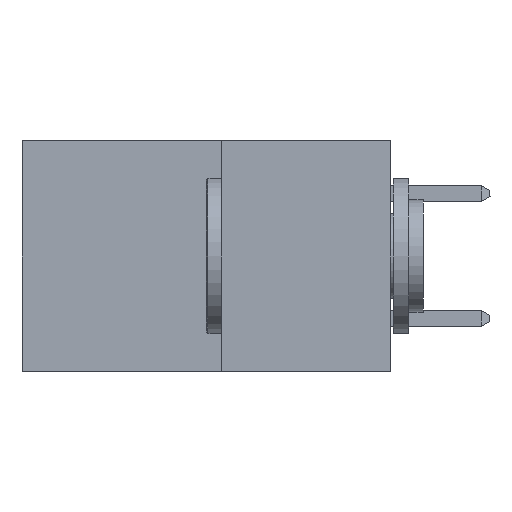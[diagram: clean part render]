
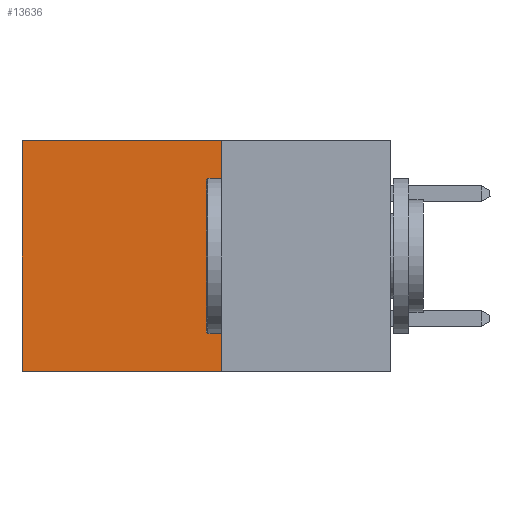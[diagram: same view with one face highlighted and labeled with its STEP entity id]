
A CAD part, left-side view. The second image highlights one B-rep face of the part: STEP entity #13636.
In plain terms, the highlighted planar face has unit normal (-1, 0, 0).
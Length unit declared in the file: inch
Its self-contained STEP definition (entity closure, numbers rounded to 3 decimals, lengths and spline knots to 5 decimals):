
#1156 = CARTESIAN_POINT ( 'NONE',  ( 0.277, 0.59, -0.37 ) ) ;
#1616 = FACE_OUTER_BOUND ( 'NONE', #6437, .T. ) ;
#2071 = CARTESIAN_POINT ( 'NONE',  ( 0.277, 0.27, -0.37 ) ) ;
#2269 = EDGE_CURVE ( 'NONE', #29836, #12502, #33518, .T. ) ;
#3433 = CARTESIAN_POINT ( 'NONE',  ( 0.277, 0.27, 0. ) ) ;
#3795 = ORIENTED_EDGE ( 'NONE', *, *, #24421, .F. ) ;
#4114 = CARTESIAN_POINT ( 'NONE',  ( 0.277, 0.27, -0.37 ) ) ;
#4438 = VECTOR ( 'NONE', #30401, 39.37008 ) ;
#4965 = VECTOR ( 'NONE', #28150, 39.37008 ) ;
#6162 = VECTOR ( 'NONE', #24502, 39.37008 ) ;
#6437 = EDGE_LOOP ( 'NONE', ( #29407, #33716, #3795, #8160 ) ) ;
#6461 = VERTEX_POINT ( 'NONE', #4114 ) ;
#8160 = ORIENTED_EDGE ( 'NONE', *, *, #19392, .T. ) ;
#8619 = CARTESIAN_POINT ( 'NONE',  ( 0.277, 0.27, 0. ) ) ;
#10377 = EDGE_CURVE ( 'NONE', #6461, #12502, #28482, .T. ) ;
#10956 = CARTESIAN_POINT ( 'NONE',  ( 0.277, 0.27, -0.37 ) ) ;
#12476 = LINE ( 'NONE', #3433, #4438 ) ;
#12502 = VERTEX_POINT ( 'NONE', #19496 ) ;
#12980 = PLANE ( 'NONE',  #24874 ) ;
#13636 = ADVANCED_FACE ( 'NONE', ( #1616 ), #12980, .F. ) ;
#15710 = DIRECTION ( 'NONE',  ( 0., 0., -1. ) ) ;
#19392 = EDGE_CURVE ( 'NONE', #23658, #29836, #12476, .T. ) ;
#19496 = CARTESIAN_POINT ( 'NONE',  ( 0.277, 0.59, -0.37 ) ) ;
#22713 = LINE ( 'NONE', #32967, #30647 ) ;
#23658 = VERTEX_POINT ( 'NONE', #8619 ) ;
#24421 = EDGE_CURVE ( 'NONE', #23658, #6461, #22713, .T. ) ;
#24502 = DIRECTION ( 'NONE',  ( 0., 1., 0. ) ) ;
#24874 = AXIS2_PLACEMENT_3D ( 'NONE', #2071, #31718, #15710 ) ;
#24881 = CARTESIAN_POINT ( 'NONE',  ( 0.277, 0.59, 0. ) ) ;
#25070 = DIRECTION ( 'NONE',  ( 0., 0., -1. ) ) ;
#28150 = DIRECTION ( 'NONE',  ( 0., 0., -1. ) ) ;
#28482 = LINE ( 'NONE', #10956, #6162 ) ;
#29407 = ORIENTED_EDGE ( 'NONE', *, *, #2269, .T. ) ;
#29836 = VERTEX_POINT ( 'NONE', #24881 ) ;
#30401 = DIRECTION ( 'NONE',  ( 0., 1., 0. ) ) ;
#30647 = VECTOR ( 'NONE', #25070, 39.37008 ) ;
#31718 = DIRECTION ( 'NONE',  ( 1., 0., 0. ) ) ;
#32967 = CARTESIAN_POINT ( 'NONE',  ( 0.277, 0.27, -0.37 ) ) ;
#33518 = LINE ( 'NONE', #1156, #4965 ) ;
#33716 = ORIENTED_EDGE ( 'NONE', *, *, #10377, .F. ) ;
